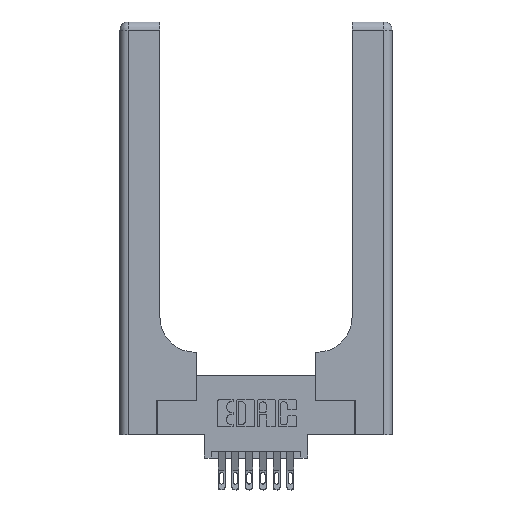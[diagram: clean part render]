
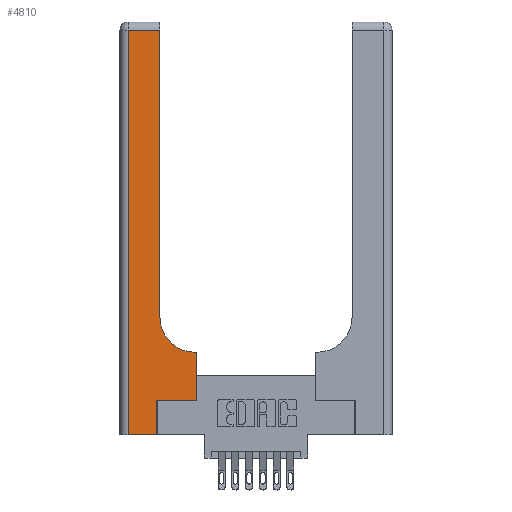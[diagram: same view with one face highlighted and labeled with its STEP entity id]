
A CAD part, top view. The second image highlights one B-rep face of the part: STEP entity #4810.
In plain terms, the highlighted planar face has unit normal (0, 0, 1).
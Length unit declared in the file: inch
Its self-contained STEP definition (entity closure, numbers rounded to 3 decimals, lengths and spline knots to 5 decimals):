
#271 = CARTESIAN_POINT ( 'NONE',  ( 0.06, 3., 0.37 ) ) ;
#301 = DIRECTION ( 'NONE',  ( 0., 1., 0. ) ) ;
#307 = DIRECTION ( 'NONE',  ( 0., -1., 0. ) ) ;
#805 = ORIENTED_EDGE ( 'NONE', *, *, #10725, .T. ) ;
#934 = VECTOR ( 'NONE', #3958, 39.37008 ) ;
#1569 = ORIENTED_EDGE ( 'NONE', *, *, #3155, .T. ) ;
#1795 = CARTESIAN_POINT ( 'NONE',  ( 0.269, 0.25, 0.37 ) ) ;
#1806 = VECTOR ( 'NONE', #6779, 39.37008 ) ;
#1870 = VECTOR ( 'NONE', #2549, 39.37008 ) ;
#2484 = DIRECTION ( 'NONE',  ( 0., 0., -1. ) ) ;
#2549 = DIRECTION ( 'NONE',  ( 0., 1., 0. ) ) ;
#2571 = ORIENTED_EDGE ( 'NONE', *, *, #5954, .T. ) ;
#2595 = ORIENTED_EDGE ( 'NONE', *, *, #8801, .T. ) ;
#3051 = DIRECTION ( 'NONE',  ( 1., 0., 0. ) ) ;
#3155 = EDGE_CURVE ( 'NONE', #13075, #14455, #13757, .T. ) ;
#3413 = ORIENTED_EDGE ( 'NONE', *, *, #5671, .T. ) ;
#3958 = DIRECTION ( 'NONE',  ( 1., 0., 0. ) ) ;
#4177 = VECTOR ( 'NONE', #307, 39.37008 ) ;
#4753 = CARTESIAN_POINT ( 'NONE',  ( 0.269, 0.25, 0.37 ) ) ;
#4810 = ADVANCED_FACE ( 'NONE', ( #11578 ), #9567, .F. ) ;
#4894 = EDGE_CURVE ( 'NONE', #5575, #9266, #10865, .T. ) ;
#5124 = AXIS2_PLACEMENT_3D ( 'NONE', #6069, #2484, #10701 ) ;
#5327 = CARTESIAN_POINT ( 'NONE',  ( 0.5585, 0.6, 0.37 ) ) ;
#5464 = LINE ( 'NONE', #7929, #14255 ) ;
#5467 = VERTEX_POINT ( 'NONE', #13065 ) ;
#5575 = VERTEX_POINT ( 'NONE', #12137 ) ;
#5598 = VERTEX_POINT ( 'NONE', #5327 ) ;
#5609 = CARTESIAN_POINT ( 'NONE',  ( 0.5585, 0.25, 0.37 ) ) ;
#5634 = DIRECTION ( 'NONE',  ( -1., 0., 0. ) ) ;
#5671 = EDGE_CURVE ( 'NONE', #5467, #13075, #5464, .T. ) ;
#5894 = VERTEX_POINT ( 'NONE', #7489 ) ;
#5919 = VECTOR ( 'NONE', #3051, 39.37008 ) ;
#5954 = EDGE_CURVE ( 'NONE', #9266, #5467, #7632, .T. ) ;
#6069 = CARTESIAN_POINT ( 'NONE',  ( 0., 3., 0.37 ) ) ;
#6155 = EDGE_CURVE ( 'NONE', #12468, #5598, #11216, .T. ) ;
#6181 = ORIENTED_EDGE ( 'NONE', *, *, #6155, .T. ) ;
#6335 = ORIENTED_EDGE ( 'NONE', *, *, #4894, .T. ) ;
#6359 = VECTOR ( 'NONE', #13786, 39.37008 ) ;
#6363 = CARTESIAN_POINT ( 'NONE',  ( 0., 0., 0.37 ) ) ;
#6423 = CARTESIAN_POINT ( 'NONE',  ( 0.5415, 0.85, 0.37 ) ) ;
#6427 = CARTESIAN_POINT ( 'NONE',  ( 0.2915, 3., 0.37 ) ) ;
#6735 = LINE ( 'NONE', #9208, #6359 ) ;
#6779 = DIRECTION ( 'NONE',  ( 0., 1., 0. ) ) ;
#7468 = AXIS2_PLACEMENT_3D ( 'NONE', #6423, #14440, #7592 ) ;
#7489 = CARTESIAN_POINT ( 'NONE',  ( 0.269, 0., 0.37 ) ) ;
#7592 = DIRECTION ( 'NONE',  ( 1., 0., 0. ) ) ;
#7632 = LINE ( 'NONE', #6427, #13343 ) ;
#7835 = ORIENTED_EDGE ( 'NONE', *, *, #9639, .T. ) ;
#7929 = CARTESIAN_POINT ( 'NONE',  ( 0., 2.94, 0.37 ) ) ;
#8103 = CARTESIAN_POINT ( 'NONE',  ( 0.06, 2.94, 0.37 ) ) ;
#8433 = ORIENTED_EDGE ( 'NONE', *, *, #13069, .T. ) ;
#8577 = LINE ( 'NONE', #10821, #1870 ) ;
#8801 = EDGE_CURVE ( 'NONE', #14707, #12468, #9006, .T. ) ;
#9006 = LINE ( 'NONE', #1795, #5919 ) ;
#9208 = CARTESIAN_POINT ( 'NONE',  ( 0.2915, 0.6, 0.37 ) ) ;
#9266 = VERTEX_POINT ( 'NONE', #10267 ) ;
#9567 = PLANE ( 'NONE',  #5124 ) ;
#9639 = EDGE_CURVE ( 'NONE', #14455, #5894, #13433, .T. ) ;
#10067 = CARTESIAN_POINT ( 'NONE',  ( 0.06, 0., 0.37 ) ) ;
#10267 = CARTESIAN_POINT ( 'NONE',  ( 0.2915, 0.85, 0.37 ) ) ;
#10701 = DIRECTION ( 'NONE',  ( -1., 0., 0. ) ) ;
#10725 = EDGE_CURVE ( 'NONE', #5894, #14707, #8577, .T. ) ;
#10821 = CARTESIAN_POINT ( 'NONE',  ( 0.269, 0., 0.37 ) ) ;
#10865 = CIRCLE ( 'NONE', #7468, 0.25 ) ;
#10908 = EDGE_LOOP ( 'NONE', ( #2571, #3413, #1569, #7835, #805, #2595, #6181, #8433, #6335 ) ) ;
#11082 = CARTESIAN_POINT ( 'NONE',  ( 0.5585, 0.25, 0.37 ) ) ;
#11216 = LINE ( 'NONE', #5609, #1806 ) ;
#11578 = FACE_OUTER_BOUND ( 'NONE', #10908, .T. ) ;
#12137 = CARTESIAN_POINT ( 'NONE',  ( 0.5415, 0.6, 0.37 ) ) ;
#12468 = VERTEX_POINT ( 'NONE', #11082 ) ;
#13065 = CARTESIAN_POINT ( 'NONE',  ( 0.2915, 2.94, 0.37 ) ) ;
#13069 = EDGE_CURVE ( 'NONE', #5598, #5575, #6735, .T. ) ;
#13075 = VERTEX_POINT ( 'NONE', #8103 ) ;
#13343 = VECTOR ( 'NONE', #301, 39.37008 ) ;
#13433 = LINE ( 'NONE', #6363, #934 ) ;
#13757 = LINE ( 'NONE', #271, #4177 ) ;
#13786 = DIRECTION ( 'NONE',  ( -1., 0., 0. ) ) ;
#14255 = VECTOR ( 'NONE', #5634, 39.37008 ) ;
#14440 = DIRECTION ( 'NONE',  ( 0., 0., -1. ) ) ;
#14455 = VERTEX_POINT ( 'NONE', #10067 ) ;
#14707 = VERTEX_POINT ( 'NONE', #4753 ) ;
